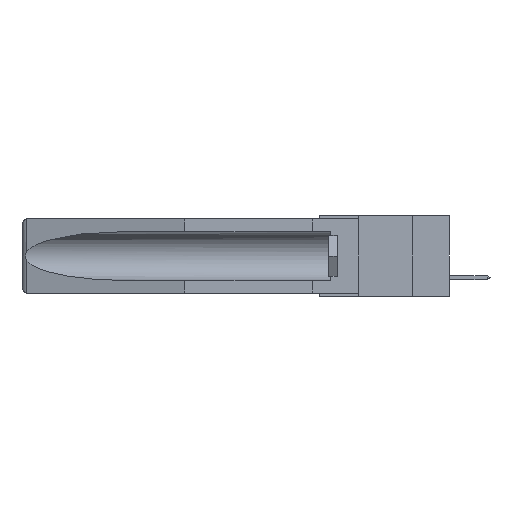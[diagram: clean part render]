
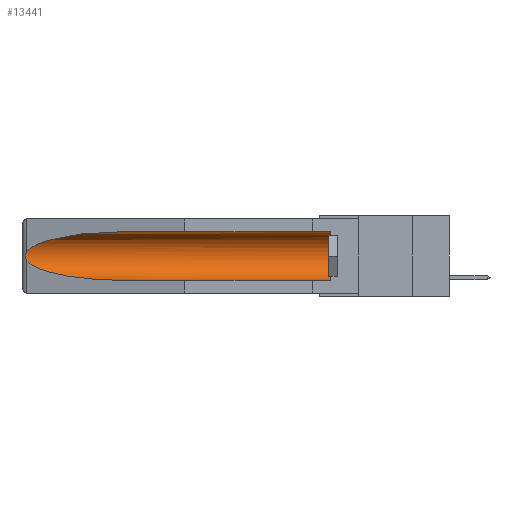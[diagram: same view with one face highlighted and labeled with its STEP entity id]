
A CAD part, left-side view. The second image highlights one B-rep face of the part: STEP entity #13441.
In plain terms, the highlighted cylindrical face has radius 2.857 mm (diameter 5.715 mm), a partial arc.
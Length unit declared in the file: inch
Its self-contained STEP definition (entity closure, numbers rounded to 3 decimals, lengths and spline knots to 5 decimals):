
#69 = CARTESIAN_POINT ( 'NONE',  ( 0.26655, 1.53094, -0.18657 ) ) ;
#160 = CARTESIAN_POINT ( 'NONE',  ( 0.2673, 1.53269, -0.17917 ) ) ;
#713 = CARTESIAN_POINT ( 'NONE',  ( 0.26654, 1.53092, -0.15636 ) ) ;
#1094 = ORIENTED_EDGE ( 'NONE', *, *, #1242, .F. ) ;
#1242 = EDGE_CURVE ( 'NONE', #21094, #2709, #9648, .T. ) ;
#1435 = CARTESIAN_POINT ( 'NONE',  ( 0.155, 0.126, -0.059 ) ) ;
#1503 = FACE_OUTER_BOUND ( 'NONE', #8618, .T. ) ;
#1595 = CARTESIAN_POINT ( 'NONE',  ( 0.155, 1.07973, -0.284 ) ) ;
#1888 = ORIENTED_EDGE ( 'NONE', *, *, #4108, .T. ) ;
#2073 = CARTESIAN_POINT ( 'NONE',  ( 0.2675, 1.53308, -0.16763 ) ) ;
#2529 = DIRECTION ( 'NONE',  ( 0., 0., 1. ) ) ;
#2709 = VERTEX_POINT ( 'NONE', #10658 ) ;
#2899 = CARTESIAN_POINT ( 'NONE',  ( 0.21114, 1.30732, -0.059 ) ) ;
#3771 = CARTESIAN_POINT ( 'NONE',  ( 0.155, 0.126, -0.1715 ) ) ;
#3998 = CARTESIAN_POINT ( 'NONE',  ( 0.26537, 1.52718, -0.14972 ) ) ;
#4108 = EDGE_CURVE ( 'NONE', #13977, #2709, #14656, .T. ) ;
#5744 = DIRECTION ( 'NONE',  ( 0., 0., 1. ) ) ;
#5890 = CARTESIAN_POINT ( 'NONE',  ( 0.26597, 1.52961, -0.15275 ) ) ;
#6975 = ORIENTED_EDGE ( 'NONE', *, *, #17249, .T. ) ;
#7229 = CARTESIAN_POINT ( 'NONE',  ( 0.21114, 1.30732, -0.284 ) ) ;
#7723 = VECTOR ( 'NONE', #10488, 39.37008 ) ;
#8281 = CARTESIAN_POINT ( 'NONE',  ( 0.155, -0.30754, -0.1715 ) ) ;
#8424 = ORIENTED_EDGE ( 'NONE', *, *, #19006, .T. ) ;
#8436 = CIRCLE ( 'NONE', #18842, 0.1125 ) ;
#8556 = B_SPLINE_CURVE_WITH_KNOTS ( 'NONE', 3,
 ( #3998, #5890, #713, #19146, #2073, #21219, #160, #69, #9799, #21141 ),
 .UNSPECIFIED., .F., .F.,
 ( 4, 2, 2, 2, 4 ),
 ( 0., 0.00029, 0.00058, 0.00087, 0.00117 ),
 .UNSPECIFIED. ) ;
#8618 = EDGE_LOOP ( 'NONE', ( #17386, #14927, #1888, #1094, #6975, #8424 ) ) ;
#9509 = CARTESIAN_POINT ( 'NONE',  ( 0.155, 1.07973, -0.059 ) ) ;
#9648 = LINE ( 'NONE', #14728, #15327 ) ;
#9799 = CARTESIAN_POINT ( 'NONE',  ( 0.26597, 1.5296, -0.19026 ) ) ;
#9834 = VERTEX_POINT ( 'NONE', #9509 ) ;
#10488 = DIRECTION ( 'NONE',  ( 0., 1., 0. ) ) ;
#10658 = CARTESIAN_POINT ( 'NONE',  ( 0.155, 1.07973, -0.284 ) ) ;
#12128 = VERTEX_POINT ( 'NONE', #1435 ) ;
#12204 = CARTESIAN_POINT ( 'NONE',  ( 0.155, -0.30754, -0.059 ) ) ;
#12831 = CARTESIAN_POINT ( 'NONE',  ( 0.25451, 1.48313, -0.09465 ) ) ;
#13280 = EDGE_CURVE ( 'NONE', #18752, #13977, #8556, .T. ) ;
#13441 = ADVANCED_FACE ( 'NONE', ( #1503 ), #14363, .F. ) ;
#13977 = VERTEX_POINT ( 'NONE', #14553 ) ;
#14363 = CYLINDRICAL_SURFACE ( 'NONE', #20209, 0.1125 ) ;
#14366 = CARTESIAN_POINT ( 'NONE',  ( 0.155, 0.126, -0.284 ) ) ;
#14547 = DIRECTION ( 'NONE',  ( 0., 1., 0. ) ) ;
#14553 = CARTESIAN_POINT ( 'NONE',  ( 0.26537, 1.52718, -0.19328 ) ) ;
#14656 =( BOUNDED_CURVE ( )  B_SPLINE_CURVE ( 3, ( #22575, #14744, #7229, #1595 ),
 .UNSPECIFIED., .F., .F. ) 
 B_SPLINE_CURVE_WITH_KNOTS ( ( 4, 4 ),
 ( 0.1948, 1.5708 ),
 .UNSPECIFIED. ) 
 CURVE ( )  GEOMETRIC_REPRESENTATION_ITEM ( )  RATIONAL_B_SPLINE_CURVE ( ( 1., 0.848, 0.848, 1. ) ) 
 REPRESENTATION_ITEM ( '' )  );
#14728 = CARTESIAN_POINT ( 'NONE',  ( 0.155, -0.30754, -0.284 ) ) ;
#14744 = CARTESIAN_POINT ( 'NONE',  ( 0.25451, 1.48313, -0.24835 ) ) ;
#14927 = ORIENTED_EDGE ( 'NONE', *, *, #13280, .T. ) ;
#15109 = DIRECTION ( 'NONE',  ( 0., -1., 0. ) ) ;
#15327 = VECTOR ( 'NONE', #14547, 39.37008 ) ;
#17249 = EDGE_CURVE ( 'NONE', #21094, #12128, #8436, .T. ) ;
#17386 = ORIENTED_EDGE ( 'NONE', *, *, #24361, .T. ) ;
#17505 = DIRECTION ( 'NONE',  ( 0., 1., 0. ) ) ;
#18752 = VERTEX_POINT ( 'NONE', #19603 ) ;
#18842 = AXIS2_PLACEMENT_3D ( 'NONE', #3771, #15109, #5744 ) ;
#19006 = EDGE_CURVE ( 'NONE', #12128, #9834, #22084, .T. ) ;
#19146 = CARTESIAN_POINT ( 'NONE',  ( 0.2673, 1.5327, -0.16383 ) ) ;
#19603 = CARTESIAN_POINT ( 'NONE',  ( 0.26537, 1.52718, -0.14972 ) ) ;
#20173 = CARTESIAN_POINT ( 'NONE',  ( 0.155, 1.07973, -0.059 ) ) ;
#20209 = AXIS2_PLACEMENT_3D ( 'NONE', #8281, #17505, #2529 ) ;
#21094 = VERTEX_POINT ( 'NONE', #14366 ) ;
#21141 = CARTESIAN_POINT ( 'NONE',  ( 0.26537, 1.52718, -0.19328 ) ) ;
#21219 = CARTESIAN_POINT ( 'NONE',  ( 0.2675, 1.53308, -0.17534 ) ) ;
#22084 = LINE ( 'NONE', #12204, #7723 ) ;
#22575 = CARTESIAN_POINT ( 'NONE',  ( 0.26537, 1.52718, -0.19328 ) ) ;
#24196 =( BOUNDED_CURVE ( )  B_SPLINE_CURVE ( 3, ( #20173, #2899, #12831, #24314 ),
 .UNSPECIFIED., .F., .F. ) 
 B_SPLINE_CURVE_WITH_KNOTS ( ( 4, 4 ),
 ( 4.71239, 6.08839 ),
 .UNSPECIFIED. ) 
 CURVE ( )  GEOMETRIC_REPRESENTATION_ITEM ( )  RATIONAL_B_SPLINE_CURVE ( ( 1., 0.848, 0.848, 1. ) ) 
 REPRESENTATION_ITEM ( '' )  );
#24314 = CARTESIAN_POINT ( 'NONE',  ( 0.26537, 1.52718, -0.14972 ) ) ;
#24361 = EDGE_CURVE ( 'NONE', #9834, #18752, #24196, .T. ) ;
